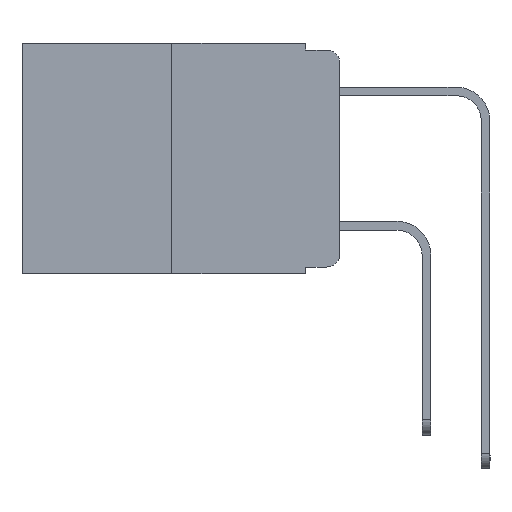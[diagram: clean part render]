
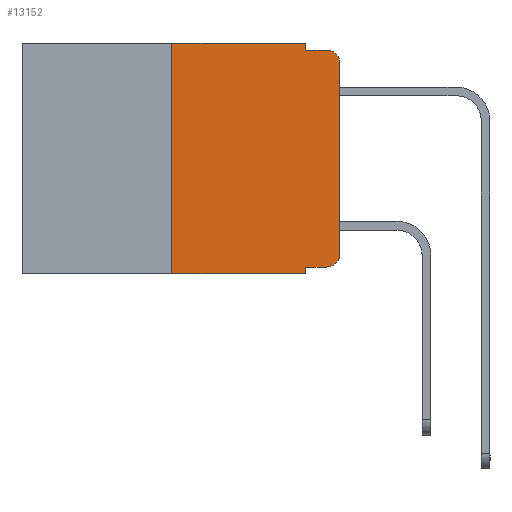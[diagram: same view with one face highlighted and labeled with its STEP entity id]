
A CAD part, left-side view. The second image highlights one B-rep face of the part: STEP entity #13152.
In plain terms, the highlighted planar face has unit normal (-1, 0, 0).
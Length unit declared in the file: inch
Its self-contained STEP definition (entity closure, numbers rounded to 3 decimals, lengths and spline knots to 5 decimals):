
#32 = ORIENTED_EDGE ( 'NONE', *, *, #7586, .F. ) ;
#284 = DIRECTION ( 'NONE',  ( 0., 0., -1. ) ) ;
#348 = LINE ( 'NONE', #10246, #12280 ) ;
#509 = VERTEX_POINT ( 'NONE', #654 ) ;
#512 = AXIS2_PLACEMENT_3D ( 'NONE', #12369, #15700, #879 ) ;
#550 = DIRECTION ( 'NONE',  ( 0., 0., -1. ) ) ;
#654 = CARTESIAN_POINT ( 'NONE',  ( 0., 0.25, -0.343 ) ) ;
#738 = EDGE_LOOP ( 'NONE', ( #15969, #12489, #32, #5099, #12811, #12480, #8299, #5601, #8186, #7204 ) ) ;
#815 = EDGE_CURVE ( 'NONE', #11016, #3966, #14489, .T. ) ;
#879 = DIRECTION ( 'NONE',  ( 0., 0., -1. ) ) ;
#1019 = EDGE_CURVE ( 'NONE', #11016, #1824, #10789, .T. ) ;
#1259 = AXIS2_PLACEMENT_3D ( 'NONE', #11459, #14061, #5093 ) ;
#1319 = VECTOR ( 'NONE', #8825, 39.37008 ) ;
#1327 = DIRECTION ( 'NONE',  ( 0., 0., 1. ) ) ;
#1727 = VECTOR ( 'NONE', #6603, 39.37008 ) ;
#1751 = VECTOR ( 'NONE', #1327, 39.37008 ) ;
#1824 = VERTEX_POINT ( 'NONE', #9209 ) ;
#2109 = VERTEX_POINT ( 'NONE', #4180 ) ;
#2505 = VECTOR ( 'NONE', #550, 39.37008 ) ;
#2508 = CARTESIAN_POINT ( 'NONE',  ( 0., 0.02, -0.333 ) ) ;
#3071 = EDGE_CURVE ( 'NONE', #2109, #3643, #348, .T. ) ;
#3390 = CARTESIAN_POINT ( 'NONE',  ( 0., 0.051, 0. ) ) ;
#3487 = AXIS2_PLACEMENT_3D ( 'NONE', #13040, #5411, #284 ) ;
#3559 = DIRECTION ( 'NONE',  ( 0., 0., 1. ) ) ;
#3643 = VERTEX_POINT ( 'NONE', #12131 ) ;
#3701 = EDGE_CURVE ( 'NONE', #3966, #8016, #7730, .T. ) ;
#3864 = EDGE_CURVE ( 'NONE', #12755, #2109, #16316, .T. ) ;
#3966 = VERTEX_POINT ( 'NONE', #2508 ) ;
#4088 = DIRECTION ( 'NONE',  ( 0., -1., 0. ) ) ;
#4180 = CARTESIAN_POINT ( 'NONE',  ( 0., 0.051, 0. ) ) ;
#4292 = CARTESIAN_POINT ( 'NONE',  ( 0., 0.473, -0.343 ) ) ;
#4552 = VERTEX_POINT ( 'NONE', #8209 ) ;
#4612 = VERTEX_POINT ( 'NONE', #14594 ) ;
#5093 = DIRECTION ( 'NONE',  ( 0., 0., -1. ) ) ;
#5099 = ORIENTED_EDGE ( 'NONE', *, *, #3071, .F. ) ;
#5285 = CARTESIAN_POINT ( 'NONE',  ( 0., 0., 0. ) ) ;
#5411 = DIRECTION ( 'NONE',  ( -1., 0., 0. ) ) ;
#5437 = CARTESIAN_POINT ( 'NONE',  ( 0., 0.051, -0.01 ) ) ;
#5452 = EDGE_CURVE ( 'NONE', #4612, #4552, #13937, .T. ) ;
#5523 = VECTOR ( 'NONE', #3559, 39.37008 ) ;
#5526 = CARTESIAN_POINT ( 'NONE',  ( 0., 0.051, -0.333 ) ) ;
#5601 = ORIENTED_EDGE ( 'NONE', *, *, #1019, .F. ) ;
#5807 = DIRECTION ( 'NONE',  ( 0., -1., 0. ) ) ;
#6603 = DIRECTION ( 'NONE',  ( 0., -1., 0. ) ) ;
#7204 = ORIENTED_EDGE ( 'NONE', *, *, #3701, .T. ) ;
#7586 = EDGE_CURVE ( 'NONE', #3643, #4552, #12739, .T. ) ;
#7588 = LINE ( 'NONE', #14050, #5523 ) ;
#7730 = CIRCLE ( 'NONE', #512, 0.02 ) ;
#8016 = VERTEX_POINT ( 'NONE', #15401 ) ;
#8186 = ORIENTED_EDGE ( 'NONE', *, *, #815, .T. ) ;
#8209 = CARTESIAN_POINT ( 'NONE',  ( 0., 0.02, -0.01 ) ) ;
#8299 = ORIENTED_EDGE ( 'NONE', *, *, #14432, .T. ) ;
#8825 = DIRECTION ( 'NONE',  ( 0., -1., 0. ) ) ;
#9113 = LINE ( 'NONE', #5285, #1751 ) ;
#9204 = CARTESIAN_POINT ( 'NONE',  ( 0., 0.051, -0.333 ) ) ;
#9209 = CARTESIAN_POINT ( 'NONE',  ( 0., 0.051, -0.343 ) ) ;
#9928 = CARTESIAN_POINT ( 'NONE',  ( 0., 0.473, 0. ) ) ;
#9974 = EDGE_CURVE ( 'NONE', #509, #12755, #7588, .T. ) ;
#10246 = CARTESIAN_POINT ( 'NONE',  ( 0., 0.051, 0. ) ) ;
#10789 = LINE ( 'NONE', #3390, #2505 ) ;
#10802 = EDGE_CURVE ( 'NONE', #8016, #4612, #9113, .T. ) ;
#10831 = LINE ( 'NONE', #4292, #12676 ) ;
#11016 = VERTEX_POINT ( 'NONE', #9204 ) ;
#11459 = CARTESIAN_POINT ( 'NONE',  ( 0., 0.473, 0. ) ) ;
#12131 = CARTESIAN_POINT ( 'NONE',  ( 0., 0.051, -0.01 ) ) ;
#12280 = VECTOR ( 'NONE', #15372, 39.37008 ) ;
#12369 = CARTESIAN_POINT ( 'NONE',  ( 0., 0.02, -0.313 ) ) ;
#12480 = ORIENTED_EDGE ( 'NONE', *, *, #9974, .F. ) ;
#12489 = ORIENTED_EDGE ( 'NONE', *, *, #5452, .T. ) ;
#12624 = PLANE ( 'NONE',  #1259 ) ;
#12676 = VECTOR ( 'NONE', #5807, 39.37008 ) ;
#12739 = LINE ( 'NONE', #5437, #12932 ) ;
#12755 = VERTEX_POINT ( 'NONE', #13919 ) ;
#12811 = ORIENTED_EDGE ( 'NONE', *, *, #3864, .F. ) ;
#12932 = VECTOR ( 'NONE', #4088, 39.37008 ) ;
#13040 = CARTESIAN_POINT ( 'NONE',  ( 0., 0.02, -0.03 ) ) ;
#13152 = ADVANCED_FACE ( 'NONE', ( #14778 ), #12624, .F. ) ;
#13919 = CARTESIAN_POINT ( 'NONE',  ( 0., 0.25, 0. ) ) ;
#13937 = CIRCLE ( 'NONE', #3487, 0.02 ) ;
#14050 = CARTESIAN_POINT ( 'NONE',  ( 0., 0.25, 0. ) ) ;
#14061 = DIRECTION ( 'NONE',  ( 1., 0., 0. ) ) ;
#14432 = EDGE_CURVE ( 'NONE', #509, #1824, #10831, .T. ) ;
#14489 = LINE ( 'NONE', #5526, #1727 ) ;
#14594 = CARTESIAN_POINT ( 'NONE',  ( 0., 0., -0.03 ) ) ;
#14778 = FACE_OUTER_BOUND ( 'NONE', #738, .T. ) ;
#15372 = DIRECTION ( 'NONE',  ( 0., 0., -1. ) ) ;
#15401 = CARTESIAN_POINT ( 'NONE',  ( 0., 0., -0.313 ) ) ;
#15700 = DIRECTION ( 'NONE',  ( -1., 0., 0. ) ) ;
#15969 = ORIENTED_EDGE ( 'NONE', *, *, #10802, .T. ) ;
#16316 = LINE ( 'NONE', #9928, #1319 ) ;
